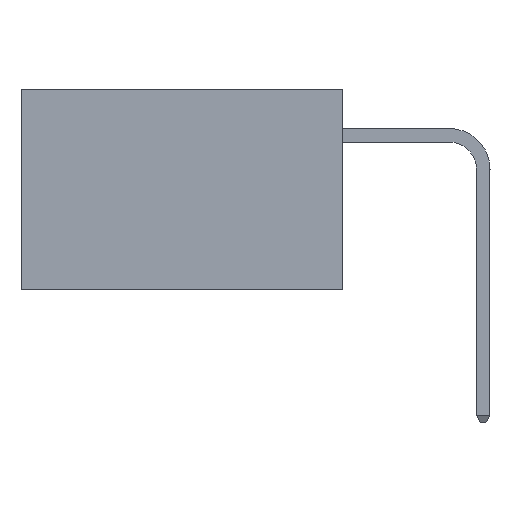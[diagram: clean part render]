
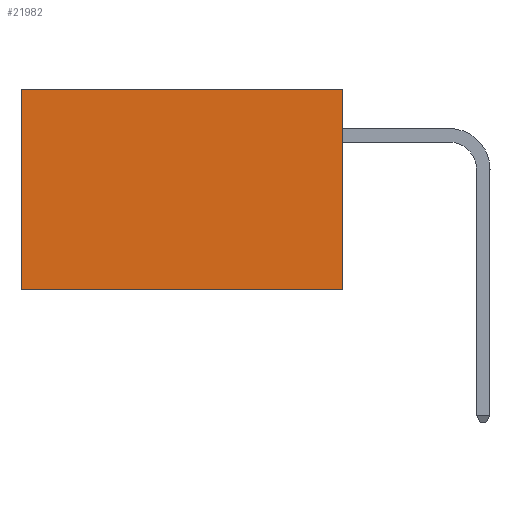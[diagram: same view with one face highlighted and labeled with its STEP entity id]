
A CAD part, left-side view. The second image highlights one B-rep face of the part: STEP entity #21982.
In plain terms, the highlighted planar face has unit normal (-1, 0, 0).
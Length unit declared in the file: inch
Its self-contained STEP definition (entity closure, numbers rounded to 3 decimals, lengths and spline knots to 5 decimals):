
#1083 = VERTEX_POINT ( 'NONE', #10568 ) ;
#1376 = VERTEX_POINT ( 'NONE', #24557 ) ;
#1946 = LINE ( 'NONE', #16277, #18680 ) ;
#2060 = DIRECTION ( 'NONE',  ( 1., 0., 0. ) ) ;
#2546 = VECTOR ( 'NONE', #23313, 39.37008 ) ;
#3492 = EDGE_CURVE ( 'NONE', #1376, #27485, #1946, .T. ) ;
#3954 = CARTESIAN_POINT ( 'NONE',  ( 0.277, 0.59, -0.37 ) ) ;
#4253 = LINE ( 'NONE', #3954, #19614 ) ;
#4836 = ORIENTED_EDGE ( 'NONE', *, *, #8159, .F. ) ;
#6055 = CARTESIAN_POINT ( 'NONE',  ( 0.277, 0.59, -0.37 ) ) ;
#7064 = VECTOR ( 'NONE', #21612, 39.37008 ) ;
#7745 = LINE ( 'NONE', #19560, #7064 ) ;
#8159 = EDGE_CURVE ( 'NONE', #1376, #1083, #7745, .T. ) ;
#8251 = CARTESIAN_POINT ( 'NONE',  ( 0.277, 0., -0.37 ) ) ;
#8389 = LINE ( 'NONE', #8251, #2546 ) ;
#8589 = PLANE ( 'NONE',  #20415 ) ;
#8746 = EDGE_CURVE ( 'NONE', #27485, #16730, #4253, .T. ) ;
#10288 = FACE_OUTER_BOUND ( 'NONE', #10807, .T. ) ;
#10568 = CARTESIAN_POINT ( 'NONE',  ( 0.277, 0., -0.37 ) ) ;
#10579 = DIRECTION ( 'NONE',  ( 0., 0., -1. ) ) ;
#10807 = EDGE_LOOP ( 'NONE', ( #11022, #18573, #4836, #10961 ) ) ;
#10961 = ORIENTED_EDGE ( 'NONE', *, *, #3492, .T. ) ;
#11022 = ORIENTED_EDGE ( 'NONE', *, *, #8746, .T. ) ;
#11254 = DIRECTION ( 'NONE',  ( 0., 1., 0. ) ) ;
#15187 = CARTESIAN_POINT ( 'NONE',  ( 0.277, 0., -0.37 ) ) ;
#16277 = CARTESIAN_POINT ( 'NONE',  ( 0.277, 0., 0. ) ) ;
#16730 = VERTEX_POINT ( 'NONE', #6055 ) ;
#17349 = DIRECTION ( 'NONE',  ( 0., 0., -1. ) ) ;
#18573 = ORIENTED_EDGE ( 'NONE', *, *, #20035, .F. ) ;
#18680 = VECTOR ( 'NONE', #11254, 39.37008 ) ;
#19560 = CARTESIAN_POINT ( 'NONE',  ( 0.277, 0., -0.37 ) ) ;
#19614 = VECTOR ( 'NONE', #10579, 39.37008 ) ;
#19918 = CARTESIAN_POINT ( 'NONE',  ( 0.277, 0.59, 0. ) ) ;
#20035 = EDGE_CURVE ( 'NONE', #1083, #16730, #8389, .T. ) ;
#20415 = AXIS2_PLACEMENT_3D ( 'NONE', #15187, #2060, #17349 ) ;
#21612 = DIRECTION ( 'NONE',  ( 0., 0., -1. ) ) ;
#21982 = ADVANCED_FACE ( 'NONE', ( #10288 ), #8589, .F. ) ;
#23313 = DIRECTION ( 'NONE',  ( 0., 1., 0. ) ) ;
#24557 = CARTESIAN_POINT ( 'NONE',  ( 0.277, 0., 0. ) ) ;
#27485 = VERTEX_POINT ( 'NONE', #19918 ) ;
